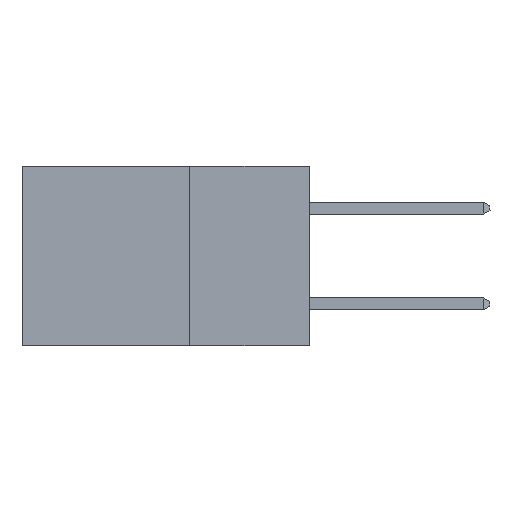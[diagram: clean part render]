
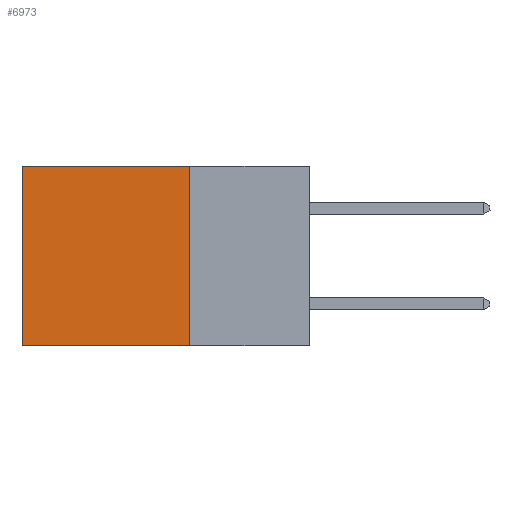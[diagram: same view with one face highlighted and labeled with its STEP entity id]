
A CAD part, left-side view. The second image highlights one B-rep face of the part: STEP entity #6973.
In plain terms, the highlighted planar face has unit normal (-1, 0, 0).
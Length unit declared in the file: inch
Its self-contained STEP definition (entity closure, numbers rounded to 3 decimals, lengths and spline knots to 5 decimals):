
#101 = DIRECTION ( 'NONE',  ( 0., 0., -1. ) ) ;
#285 = CARTESIAN_POINT ( 'NONE',  ( 0.2875, 0.25, -0.375 ) ) ;
#288 = ORIENTED_EDGE ( 'NONE', *, *, #555, .F. ) ;
#296 = DIRECTION ( 'NONE',  ( 0., 1., 0. ) ) ;
#321 = DIRECTION ( 'NONE',  ( 0., 0., -1. ) ) ;
#396 = ORIENTED_EDGE ( 'NONE', *, *, #7995, .F. ) ;
#432 = ORIENTED_EDGE ( 'NONE', *, *, #4225, .T. ) ;
#555 = EDGE_CURVE ( 'NONE', #7618, #6969, #6949, .T. ) ;
#651 = VECTOR ( 'NONE', #5193, 39.37008 ) ;
#818 = CARTESIAN_POINT ( 'NONE',  ( 0.2875, 0.25, -0.375 ) ) ;
#886 = VERTEX_POINT ( 'NONE', #3958 ) ;
#899 = VERTEX_POINT ( 'NONE', #1247 ) ;
#1247 = CARTESIAN_POINT ( 'NONE',  ( 0.2875, 0.25, 0. ) ) ;
#1527 = LINE ( 'NONE', #5635, #7475 ) ;
#1627 = CARTESIAN_POINT ( 'NONE',  ( 0.2875, 0.25, -0.375 ) ) ;
#2077 = DIRECTION ( 'NONE',  ( 1., 0., 0. ) ) ;
#2794 = CARTESIAN_POINT ( 'NONE',  ( 0.2875, 0.6, -0.375 ) ) ;
#2959 = FACE_OUTER_BOUND ( 'NONE', #6422, .T. ) ;
#3958 = CARTESIAN_POINT ( 'NONE',  ( 0.2875, 0.6, 0. ) ) ;
#4032 = VECTOR ( 'NONE', #4124, 39.37008 ) ;
#4124 = DIRECTION ( 'NONE',  ( 0., 1., 0. ) ) ;
#4225 = EDGE_CURVE ( 'NONE', #886, #6969, #6733, .T. ) ;
#5193 = DIRECTION ( 'NONE',  ( 0., 0., -1. ) ) ;
#5282 = CARTESIAN_POINT ( 'NONE',  ( 0.2875, 0.6, -0.375 ) ) ;
#5364 = CARTESIAN_POINT ( 'NONE',  ( 0.2875, 0.25, 0. ) ) ;
#5635 = CARTESIAN_POINT ( 'NONE',  ( 0.2875, 0.25, -0.375 ) ) ;
#5710 = VECTOR ( 'NONE', #296, 39.37008 ) ;
#6376 = EDGE_CURVE ( 'NONE', #899, #886, #8155, .T. ) ;
#6422 = EDGE_LOOP ( 'NONE', ( #432, #288, #396, #6500 ) ) ;
#6500 = ORIENTED_EDGE ( 'NONE', *, *, #6376, .T. ) ;
#6733 = LINE ( 'NONE', #5282, #651 ) ;
#6949 = LINE ( 'NONE', #1627, #5710 ) ;
#6969 = VERTEX_POINT ( 'NONE', #2794 ) ;
#6973 = ADVANCED_FACE ( 'NONE', ( #2959 ), #7234, .F. ) ;
#6984 = AXIS2_PLACEMENT_3D ( 'NONE', #818, #2077, #101 ) ;
#7234 = PLANE ( 'NONE',  #6984 ) ;
#7475 = VECTOR ( 'NONE', #321, 39.37008 ) ;
#7618 = VERTEX_POINT ( 'NONE', #285 ) ;
#7995 = EDGE_CURVE ( 'NONE', #899, #7618, #1527, .T. ) ;
#8155 = LINE ( 'NONE', #5364, #4032 ) ;
